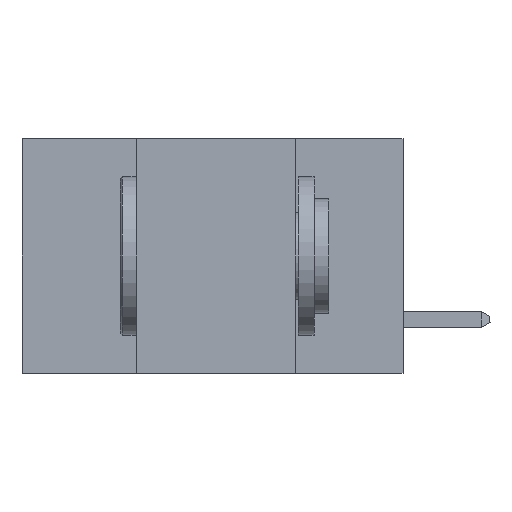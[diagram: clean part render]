
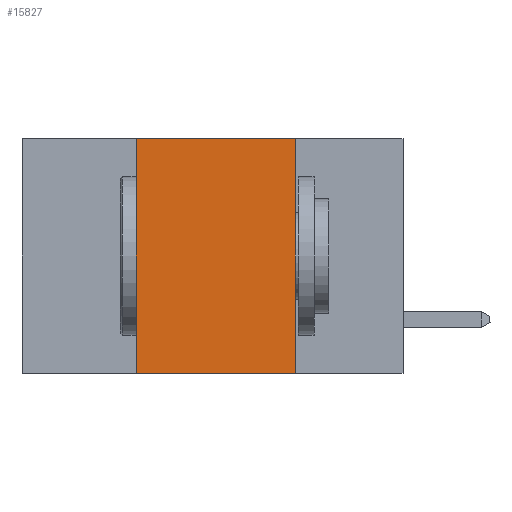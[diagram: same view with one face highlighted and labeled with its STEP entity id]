
A CAD part, left-side view. The second image highlights one B-rep face of the part: STEP entity #15827.
In plain terms, the highlighted planar face has unit normal (-1, 0, 0).
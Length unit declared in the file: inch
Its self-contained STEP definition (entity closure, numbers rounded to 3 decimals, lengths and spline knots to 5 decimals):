
#2482 = CARTESIAN_POINT ( 'NONE',  ( 0., 0.6, 0. ) ) ;
#2486 = AXIS2_PLACEMENT_3D ( 'NONE', #7316, #30681, #35254 ) ;
#3918 = PLANE ( 'NONE',  #2486 ) ;
#4159 = VECTOR ( 'NONE', #34401, 39.37008 ) ;
#6962 = DIRECTION ( 'NONE',  ( 0., 0., -1. ) ) ;
#7316 = CARTESIAN_POINT ( 'NONE',  ( 0., 0.6, 0. ) ) ;
#9026 = CARTESIAN_POINT ( 'NONE',  ( 0., 0.6, -0.37 ) ) ;
#10491 = VECTOR ( 'NONE', #6962, 39.37008 ) ;
#10772 = EDGE_CURVE ( 'NONE', #14787, #27852, #14123, .T. ) ;
#12774 = ORIENTED_EDGE ( 'NONE', *, *, #10772, .F. ) ;
#14123 = LINE ( 'NONE', #2482, #4159 ) ;
#14787 = VERTEX_POINT ( 'NONE', #25051 ) ;
#15568 = DIRECTION ( 'NONE',  ( 0., -1., 0. ) ) ;
#15827 = ADVANCED_FACE ( 'NONE', ( #26003 ), #3918, .F. ) ;
#16470 = EDGE_CURVE ( 'NONE', #19725, #25280, #33775, .T. ) ;
#16733 = CARTESIAN_POINT ( 'NONE',  ( 0., 0.17, 0. ) ) ;
#17189 = EDGE_CURVE ( 'NONE', #19725, #14787, #25429, .T. ) ;
#18444 = ORIENTED_EDGE ( 'NONE', *, *, #30619, .F. ) ;
#19725 = VERTEX_POINT ( 'NONE', #42877 ) ;
#21958 = LINE ( 'NONE', #16733, #10491 ) ;
#25051 = CARTESIAN_POINT ( 'NONE',  ( 0., 0.42, 0. ) ) ;
#25280 = VERTEX_POINT ( 'NONE', #40983 ) ;
#25429 = LINE ( 'NONE', #25927, #41204 ) ;
#25927 = CARTESIAN_POINT ( 'NONE',  ( 0., 0.42, 0. ) ) ;
#26003 = FACE_OUTER_BOUND ( 'NONE', #37473, .T. ) ;
#27852 = VERTEX_POINT ( 'NONE', #37411 ) ;
#29273 = DIRECTION ( 'NONE',  ( 0., 0., 1. ) ) ;
#30619 = EDGE_CURVE ( 'NONE', #27852, #25280, #21958, .T. ) ;
#30681 = DIRECTION ( 'NONE',  ( 1., 0., 0. ) ) ;
#33775 = LINE ( 'NONE', #9026, #34826 ) ;
#34401 = DIRECTION ( 'NONE',  ( 0., -1., 0. ) ) ;
#34826 = VECTOR ( 'NONE', #15568, 39.37008 ) ;
#35252 = ORIENTED_EDGE ( 'NONE', *, *, #17189, .F. ) ;
#35254 = DIRECTION ( 'NONE',  ( 0., 0., -1. ) ) ;
#37411 = CARTESIAN_POINT ( 'NONE',  ( 0., 0.17, 0. ) ) ;
#37473 = EDGE_LOOP ( 'NONE', ( #18444, #12774, #35252, #41474 ) ) ;
#40983 = CARTESIAN_POINT ( 'NONE',  ( 0., 0.17, -0.37 ) ) ;
#41204 = VECTOR ( 'NONE', #29273, 39.37008 ) ;
#41474 = ORIENTED_EDGE ( 'NONE', *, *, #16470, .T. ) ;
#42877 = CARTESIAN_POINT ( 'NONE',  ( 0., 0.42, -0.37 ) ) ;
